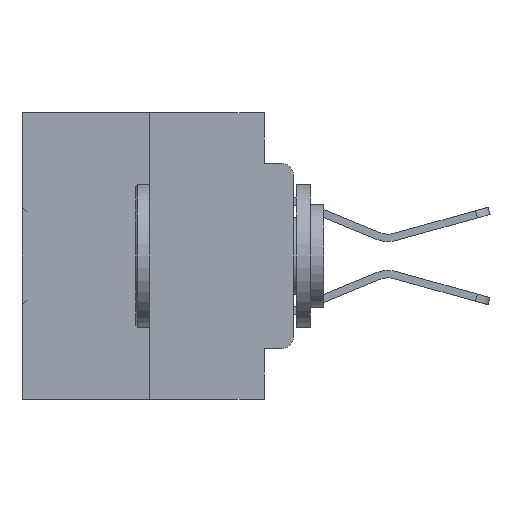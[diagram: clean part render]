
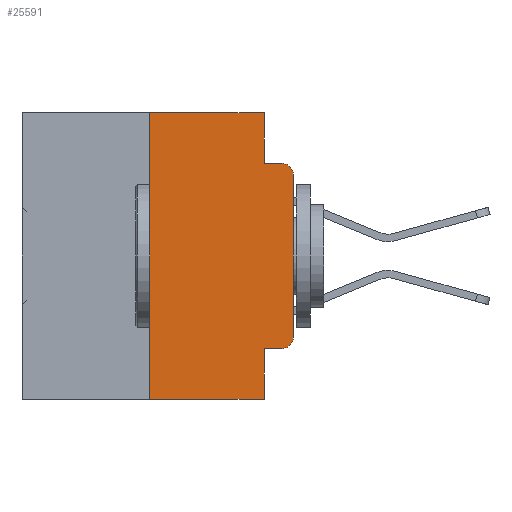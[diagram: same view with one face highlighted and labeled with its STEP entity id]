
A CAD part, left-side view. The second image highlights one B-rep face of the part: STEP entity #25591.
In plain terms, the highlighted planar face has unit normal (-1, 0, 0).
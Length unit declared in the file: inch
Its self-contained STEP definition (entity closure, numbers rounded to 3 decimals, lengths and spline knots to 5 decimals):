
#425 = EDGE_CURVE ( 'NONE', #31074, #21338, #2693, .T. ) ;
#690 = CARTESIAN_POINT ( 'NONE',  ( 0., 0.051, 0. ) ) ;
#714 = CARTESIAN_POINT ( 'NONE',  ( 0., 0.051, -0.0885 ) ) ;
#1908 = VERTEX_POINT ( 'NONE', #26426 ) ;
#2211 = LINE ( 'NONE', #35776, #4605 ) ;
#2359 = VECTOR ( 'NONE', #22389, 39.37008 ) ;
#2693 = LINE ( 'NONE', #28029, #21566 ) ;
#3984 = VERTEX_POINT ( 'NONE', #27138 ) ;
#4472 = EDGE_CURVE ( 'NONE', #3984, #19295, #13187, .T. ) ;
#4605 = VECTOR ( 'NONE', #26820, 39.37008 ) ;
#6042 = LINE ( 'NONE', #714, #33011 ) ;
#6199 = DIRECTION ( 'NONE',  ( 0., 0., -1. ) ) ;
#6624 = CARTESIAN_POINT ( 'NONE',  ( 0., 0., -0.1085 ) ) ;
#7734 = VERTEX_POINT ( 'NONE', #9313 ) ;
#8124 = ORIENTED_EDGE ( 'NONE', *, *, #28435, .T. ) ;
#8346 = DIRECTION ( 'NONE',  ( 0., -1., 0. ) ) ;
#8626 = DIRECTION ( 'NONE',  ( 0., -1., 0. ) ) ;
#8740 = ORIENTED_EDGE ( 'NONE', *, *, #11521, .T. ) ;
#8841 = EDGE_CURVE ( 'NONE', #1908, #7734, #2211, .T. ) ;
#9166 = VECTOR ( 'NONE', #35383, 39.37008 ) ;
#9265 = VECTOR ( 'NONE', #35516, 39.37008 ) ;
#9313 = CARTESIAN_POINT ( 'NONE',  ( 0., 0.25, 0. ) ) ;
#9660 = AXIS2_PLACEMENT_3D ( 'NONE', #32032, #18100, #29289 ) ;
#10272 = CIRCLE ( 'NONE', #9660, 0.02 ) ;
#11200 = CARTESIAN_POINT ( 'NONE',  ( 0., 0.473, -0.5 ) ) ;
#11521 = EDGE_CURVE ( 'NONE', #1908, #19295, #36115, .T. ) ;
#12868 = LINE ( 'NONE', #21117, #9166 ) ;
#13187 = LINE ( 'NONE', #24368, #9265 ) ;
#13549 = EDGE_CURVE ( 'NONE', #7734, #32974, #33476, .T. ) ;
#14426 = ORIENTED_EDGE ( 'NONE', *, *, #4472, .F. ) ;
#15616 = VERTEX_POINT ( 'NONE', #19258 ) ;
#16311 = DIRECTION ( 'NONE',  ( 0., 0., 1. ) ) ;
#17876 = EDGE_CURVE ( 'NONE', #15616, #31074, #10272, .T. ) ;
#17979 = ORIENTED_EDGE ( 'NONE', *, *, #20142, .F. ) ;
#18100 = DIRECTION ( 'NONE',  ( -1., 0., 0. ) ) ;
#18275 = CARTESIAN_POINT ( 'NONE',  ( 0., 0.051, -0.0885 ) ) ;
#18287 = CARTESIAN_POINT ( 'NONE',  ( 0., 0.02, -0.0885 ) ) ;
#18843 = ORIENTED_EDGE ( 'NONE', *, *, #36023, .F. ) ;
#19258 = CARTESIAN_POINT ( 'NONE',  ( 0., 0.02, -0.4115 ) ) ;
#19295 = VERTEX_POINT ( 'NONE', #27070 ) ;
#19551 = CARTESIAN_POINT ( 'NONE',  ( 0., 0.051, -0.4115 ) ) ;
#19739 = LINE ( 'NONE', #19551, #22823 ) ;
#20142 = EDGE_CURVE ( 'NONE', #32974, #21050, #12868, .T. ) ;
#20165 = CARTESIAN_POINT ( 'NONE',  ( 0., 0.473, 0. ) ) ;
#21050 = VERTEX_POINT ( 'NONE', #18275 ) ;
#21117 = CARTESIAN_POINT ( 'NONE',  ( 0., 0.051, 0. ) ) ;
#21338 = VERTEX_POINT ( 'NONE', #6624 ) ;
#21566 = VECTOR ( 'NONE', #16311, 39.37008 ) ;
#21861 = AXIS2_PLACEMENT_3D ( 'NONE', #23625, #31693, #29298 ) ;
#22232 = ORIENTED_EDGE ( 'NONE', *, *, #17876, .T. ) ;
#22389 = DIRECTION ( 'NONE',  ( 0., -1., 0. ) ) ;
#22553 = FACE_OUTER_BOUND ( 'NONE', #25229, .T. ) ;
#22823 = VECTOR ( 'NONE', #30921, 39.37008 ) ;
#23625 = CARTESIAN_POINT ( 'NONE',  ( 0., 0.02, -0.1085 ) ) ;
#24368 = CARTESIAN_POINT ( 'NONE',  ( 0., 0.051, 0. ) ) ;
#24380 = ORIENTED_EDGE ( 'NONE', *, *, #425, .T. ) ;
#24593 = EDGE_CURVE ( 'NONE', #3984, #15616, #19739, .T. ) ;
#25054 = CARTESIAN_POINT ( 'NONE',  ( 0., 0.473, 0. ) ) ;
#25219 = ORIENTED_EDGE ( 'NONE', *, *, #8841, .F. ) ;
#25229 = EDGE_LOOP ( 'NONE', ( #24380, #8124, #18843, #17979, #34800, #25219, #8740, #14426, #32147, #22232 ) ) ;
#25591 = ADVANCED_FACE ( 'NONE', ( #22553 ), #34080, .F. ) ;
#26426 = CARTESIAN_POINT ( 'NONE',  ( 0., 0.25, -0.5 ) ) ;
#26820 = DIRECTION ( 'NONE',  ( 0., 0., 1. ) ) ;
#27070 = CARTESIAN_POINT ( 'NONE',  ( 0., 0.051, -0.5 ) ) ;
#27138 = CARTESIAN_POINT ( 'NONE',  ( 0., 0.051, -0.4115 ) ) ;
#27568 = CARTESIAN_POINT ( 'NONE',  ( 0., 0., -0.3915 ) ) ;
#28029 = CARTESIAN_POINT ( 'NONE',  ( 0., 0., 0. ) ) ;
#28435 = EDGE_CURVE ( 'NONE', #21338, #28730, #32973, .T. ) ;
#28730 = VERTEX_POINT ( 'NONE', #18287 ) ;
#28744 = AXIS2_PLACEMENT_3D ( 'NONE', #20165, #31345, #6199 ) ;
#29289 = DIRECTION ( 'NONE',  ( 0., 0., -1. ) ) ;
#29298 = DIRECTION ( 'NONE',  ( 0., 0., -1. ) ) ;
#29430 = VECTOR ( 'NONE', #8346, 39.37008 ) ;
#30921 = DIRECTION ( 'NONE',  ( 0., -1., 0. ) ) ;
#31074 = VERTEX_POINT ( 'NONE', #27568 ) ;
#31345 = DIRECTION ( 'NONE',  ( 1., 0., 0. ) ) ;
#31693 = DIRECTION ( 'NONE',  ( -1., 0., 0. ) ) ;
#32032 = CARTESIAN_POINT ( 'NONE',  ( 0., 0.02, -0.3915 ) ) ;
#32147 = ORIENTED_EDGE ( 'NONE', *, *, #24593, .T. ) ;
#32974 = VERTEX_POINT ( 'NONE', #690 ) ;
#32973 = CIRCLE ( 'NONE', #21861, 0.02 ) ;
#33011 = VECTOR ( 'NONE', #8626, 39.37008 ) ;
#33476 = LINE ( 'NONE', #25054, #29430 ) ;
#34080 = PLANE ( 'NONE',  #28744 ) ;
#34800 = ORIENTED_EDGE ( 'NONE', *, *, #13549, .F. ) ;
#35383 = DIRECTION ( 'NONE',  ( 0., 0., -1. ) ) ;
#35516 = DIRECTION ( 'NONE',  ( 0., 0., -1. ) ) ;
#35776 = CARTESIAN_POINT ( 'NONE',  ( 0., 0.25, 0. ) ) ;
#36023 = EDGE_CURVE ( 'NONE', #21050, #28730, #6042, .T. ) ;
#36115 = LINE ( 'NONE', #11200, #2359 ) ;
